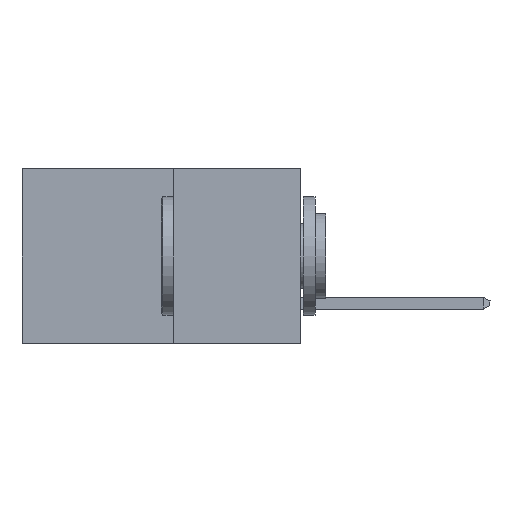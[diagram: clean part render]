
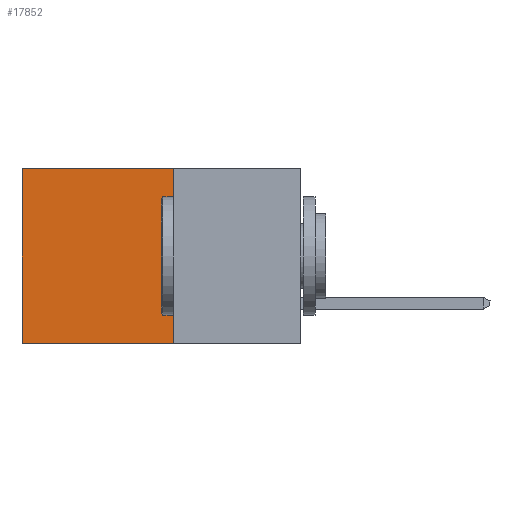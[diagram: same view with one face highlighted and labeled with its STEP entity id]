
A CAD part, left-side view. The second image highlights one B-rep face of the part: STEP entity #17852.
In plain terms, the highlighted planar face has unit normal (-1, 0, 0).
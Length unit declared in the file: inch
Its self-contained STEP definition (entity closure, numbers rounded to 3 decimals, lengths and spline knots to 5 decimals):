
#61 = DIRECTION ( 'NONE',  ( 0., 0., -1. ) ) ;
#869 = LINE ( 'NONE', #19361, #18140 ) ;
#3578 = ORIENTED_EDGE ( 'NONE', *, *, #11744, .F. ) ;
#4749 = VECTOR ( 'NONE', #22169, 39.37008 ) ;
#5313 = LINE ( 'NONE', #17061, #4749 ) ;
#7895 = VERTEX_POINT ( 'NONE', #20862 ) ;
#8078 = DIRECTION ( 'NONE',  ( 1., 0., 0. ) ) ;
#9000 = CARTESIAN_POINT ( 'NONE',  ( 0.277, 0.27, -0.37 ) ) ;
#10232 = VERTEX_POINT ( 'NONE', #18379 ) ;
#11166 = VERTEX_POINT ( 'NONE', #9000 ) ;
#11421 = EDGE_CURVE ( 'NONE', #21834, #7895, #11827, .T. ) ;
#11453 = DIRECTION ( 'NONE',  ( 0., 1., 0. ) ) ;
#11744 = EDGE_CURVE ( 'NONE', #11166, #10232, #869, .T. ) ;
#11827 = LINE ( 'NONE', #18456, #15962 ) ;
#12473 = CARTESIAN_POINT ( 'NONE',  ( 0.277, 0.59, -0.37 ) ) ;
#12962 = LINE ( 'NONE', #12473, #21692 ) ;
#13840 = ORIENTED_EDGE ( 'NONE', *, *, #22073, .T. ) ;
#14527 = FACE_OUTER_BOUND ( 'NONE', #20074, .T. ) ;
#15962 = VECTOR ( 'NONE', #11453, 39.37008 ) ;
#16012 = ORIENTED_EDGE ( 'NONE', *, *, #17232, .F. ) ;
#17061 = CARTESIAN_POINT ( 'NONE',  ( 0.277, 0.27, -0.37 ) ) ;
#17121 = CARTESIAN_POINT ( 'NONE',  ( 0.277, 0.27, 0. ) ) ;
#17232 = EDGE_CURVE ( 'NONE', #21834, #11166, #5313, .T. ) ;
#17852 = ADVANCED_FACE ( 'NONE', ( #14527 ), #18718, .F. ) ;
#18140 = VECTOR ( 'NONE', #21073, 39.37008 ) ;
#18379 = CARTESIAN_POINT ( 'NONE',  ( 0.277, 0.59, -0.37 ) ) ;
#18456 = CARTESIAN_POINT ( 'NONE',  ( 0.277, 0.27, 0. ) ) ;
#18718 = PLANE ( 'NONE',  #19272 ) ;
#19183 = ORIENTED_EDGE ( 'NONE', *, *, #11421, .T. ) ;
#19272 = AXIS2_PLACEMENT_3D ( 'NONE', #20379, #8078, #20454 ) ;
#19361 = CARTESIAN_POINT ( 'NONE',  ( 0.277, 0.27, -0.37 ) ) ;
#20074 = EDGE_LOOP ( 'NONE', ( #13840, #3578, #16012, #19183 ) ) ;
#20379 = CARTESIAN_POINT ( 'NONE',  ( 0.277, 0.27, -0.37 ) ) ;
#20454 = DIRECTION ( 'NONE',  ( 0., 0., -1. ) ) ;
#20862 = CARTESIAN_POINT ( 'NONE',  ( 0.277, 0.59, 0. ) ) ;
#21073 = DIRECTION ( 'NONE',  ( 0., 1., 0. ) ) ;
#21692 = VECTOR ( 'NONE', #61, 39.37008 ) ;
#21834 = VERTEX_POINT ( 'NONE', #17121 ) ;
#22073 = EDGE_CURVE ( 'NONE', #7895, #10232, #12962, .T. ) ;
#22169 = DIRECTION ( 'NONE',  ( 0., 0., -1. ) ) ;
